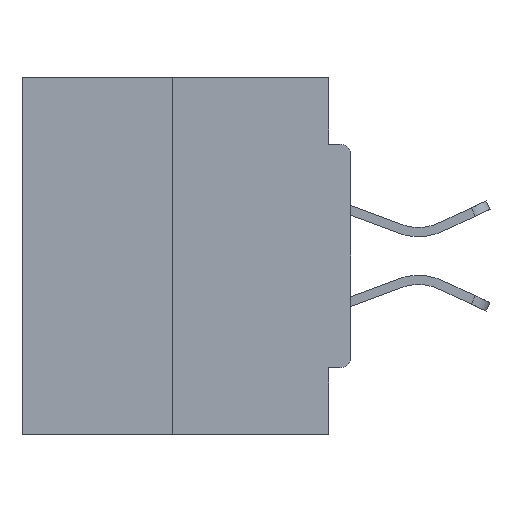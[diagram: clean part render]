
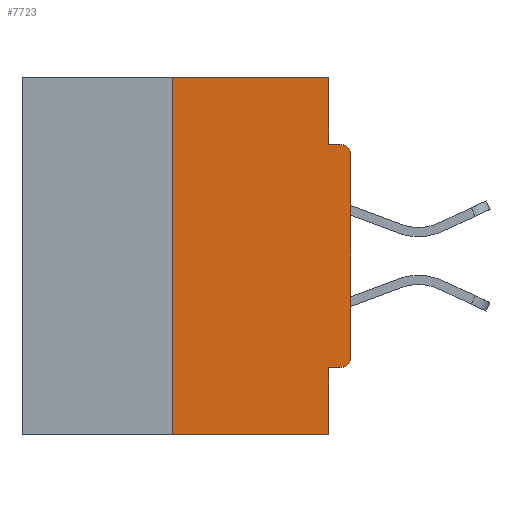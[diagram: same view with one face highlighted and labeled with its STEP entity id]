
A CAD part, left-side view. The second image highlights one B-rep face of the part: STEP entity #7723.
In plain terms, the highlighted planar face has unit normal (-1, 0, 0).
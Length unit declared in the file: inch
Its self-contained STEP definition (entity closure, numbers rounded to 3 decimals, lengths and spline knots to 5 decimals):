
#159 = VERTEX_POINT ( 'NONE', #36421 ) ;
#438 = VERTEX_POINT ( 'NONE', #6405 ) ;
#463 = DIRECTION ( 'NONE',  ( 0., 0., -1. ) ) ;
#654 = CARTESIAN_POINT ( 'NONE',  ( 0., 0., 0. ) ) ;
#776 = LINE ( 'NONE', #13028, #17385 ) ;
#2777 = CARTESIAN_POINT ( 'NONE',  ( 0., 0., -0.0935 ) ) ;
#3005 = ORIENTED_EDGE ( 'NONE', *, *, #11192, .F. ) ;
#3043 = ORIENTED_EDGE ( 'NONE', *, *, #33751, .F. ) ;
#3089 = CARTESIAN_POINT ( 'NONE',  ( 0., 0.031, 0. ) ) ;
#3435 = ORIENTED_EDGE ( 'NONE', *, *, #31251, .F. ) ;
#3451 = DIRECTION ( 'NONE',  ( -1., 0., 0. ) ) ;
#5044 = VECTOR ( 'NONE', #34973, 39.37008 ) ;
#6065 = VECTOR ( 'NONE', #16706, 39.37008 ) ;
#6351 = DIRECTION ( 'NONE',  ( 1., 0., 0. ) ) ;
#6405 = CARTESIAN_POINT ( 'NONE',  ( 0., 0.031, -0.0935 ) ) ;
#6429 = EDGE_CURVE ( 'NONE', #27034, #14101, #776, .T. ) ;
#6594 = AXIS2_PLACEMENT_3D ( 'NONE', #17671, #8720, #463 ) ;
#6656 = ORIENTED_EDGE ( 'NONE', *, *, #34932, .F. ) ;
#6837 = VERTEX_POINT ( 'NONE', #12852 ) ;
#7429 = ORIENTED_EDGE ( 'NONE', *, *, #32899, .T. ) ;
#7723 = ADVANCED_FACE ( 'NONE', ( #20023 ), #23178, .F. ) ;
#7780 = EDGE_CURVE ( 'NONE', #6837, #30905, #22709, .T. ) ;
#8025 = CARTESIAN_POINT ( 'NONE',  ( 0., 0.031, 0. ) ) ;
#8124 = VECTOR ( 'NONE', #19732, 39.37008 ) ;
#8354 = CARTESIAN_POINT ( 'NONE',  ( 0., 0.25, 0. ) ) ;
#8720 = DIRECTION ( 'NONE',  ( -1., 0., 0. ) ) ;
#8802 = CARTESIAN_POINT ( 'NONE',  ( 0., 0.46, -0.5 ) ) ;
#9213 = EDGE_CURVE ( 'NONE', #13541, #30361, #21698, .T. ) ;
#10142 = ORIENTED_EDGE ( 'NONE', *, *, #28367, .F. ) ;
#10775 = CARTESIAN_POINT ( 'NONE',  ( 0., 0.25, 0. ) ) ;
#10821 = EDGE_LOOP ( 'NONE', ( #23040, #6656, #7429, #3435, #3005, #33921, #20419, #21114, #3043, #10142 ) ) ;
#11024 = LINE ( 'NONE', #8802, #32306 ) ;
#11192 = EDGE_CURVE ( 'NONE', #13541, #24240, #19266, .T. ) ;
#11723 = DIRECTION ( 'NONE',  ( 0., 0., -1. ) ) ;
#12223 = CARTESIAN_POINT ( 'NONE',  ( 0., 0.031, -0.5 ) ) ;
#12396 = CARTESIAN_POINT ( 'NONE',  ( 0., 0.015, -0.0935 ) ) ;
#12852 = CARTESIAN_POINT ( 'NONE',  ( 0., 0., -0.1085 ) ) ;
#12979 = CARTESIAN_POINT ( 'NONE',  ( 0., 0.031, -0.4065 ) ) ;
#13028 = CARTESIAN_POINT ( 'NONE',  ( 0., 0.46, 0. ) ) ;
#13541 = VERTEX_POINT ( 'NONE', #21188 ) ;
#14094 = CARTESIAN_POINT ( 'NONE',  ( 0., 0., -0.4065 ) ) ;
#14101 = VERTEX_POINT ( 'NONE', #8025 ) ;
#14108 = LINE ( 'NONE', #2777, #6065 ) ;
#16706 = DIRECTION ( 'NONE',  ( 0., -1., 0. ) ) ;
#17037 = VECTOR ( 'NONE', #35684, 39.37008 ) ;
#17251 = DIRECTION ( 'NONE',  ( 0., -1., 0. ) ) ;
#17385 = VECTOR ( 'NONE', #33639, 39.37008 ) ;
#17671 = CARTESIAN_POINT ( 'NONE',  ( 0., 0.015, -0.1085 ) ) ;
#19266 = LINE ( 'NONE', #14094, #17037 ) ;
#19732 = DIRECTION ( 'NONE',  ( 0., 0., 1. ) ) ;
#20023 = FACE_OUTER_BOUND ( 'NONE', #10821, .T. ) ;
#20419 = ORIENTED_EDGE ( 'NONE', *, *, #22664, .T. ) ;
#20797 = AXIS2_PLACEMENT_3D ( 'NONE', #35104, #6351, #11723 ) ;
#20971 = DIRECTION ( 'NONE',  ( 0., 0., 1. ) ) ;
#21114 = ORIENTED_EDGE ( 'NONE', *, *, #7780, .T. ) ;
#21188 = CARTESIAN_POINT ( 'NONE',  ( 0., 0.015, -0.4065 ) ) ;
#21698 = CIRCLE ( 'NONE', #24425, 0.015 ) ;
#21889 = VECTOR ( 'NONE', #20971, 39.37008 ) ;
#22664 = EDGE_CURVE ( 'NONE', #30361, #6837, #31887, .T. ) ;
#22709 = CIRCLE ( 'NONE', #6594, 0.015 ) ;
#23040 = ORIENTED_EDGE ( 'NONE', *, *, #6429, .F. ) ;
#23178 = PLANE ( 'NONE',  #20797 ) ;
#23322 = VECTOR ( 'NONE', #32589, 39.37008 ) ;
#24173 = VERTEX_POINT ( 'NONE', #27129 ) ;
#24240 = VERTEX_POINT ( 'NONE', #12979 ) ;
#24425 = AXIS2_PLACEMENT_3D ( 'NONE', #34839, #3451, #26453 ) ;
#25134 = LINE ( 'NONE', #12223, #23322 ) ;
#26453 = DIRECTION ( 'NONE',  ( 0., 0., -1. ) ) ;
#27034 = VERTEX_POINT ( 'NONE', #8354 ) ;
#27129 = CARTESIAN_POINT ( 'NONE',  ( 0., 0.031, -0.5 ) ) ;
#27521 = LINE ( 'NONE', #3089, #5044 ) ;
#28367 = EDGE_CURVE ( 'NONE', #14101, #438, #27521, .T. ) ;
#28718 = CARTESIAN_POINT ( 'NONE',  ( 0., 0., -0.3915 ) ) ;
#30361 = VERTEX_POINT ( 'NONE', #28718 ) ;
#30905 = VERTEX_POINT ( 'NONE', #12396 ) ;
#31134 = LINE ( 'NONE', #10775, #8124 ) ;
#31251 = EDGE_CURVE ( 'NONE', #24240, #24173, #25134, .T. ) ;
#31887 = LINE ( 'NONE', #654, #21889 ) ;
#32306 = VECTOR ( 'NONE', #17251, 39.37008 ) ;
#32589 = DIRECTION ( 'NONE',  ( 0., 0., -1. ) ) ;
#32899 = EDGE_CURVE ( 'NONE', #159, #24173, #11024, .T. ) ;
#33639 = DIRECTION ( 'NONE',  ( 0., -1., 0. ) ) ;
#33751 = EDGE_CURVE ( 'NONE', #438, #30905, #14108, .T. ) ;
#33921 = ORIENTED_EDGE ( 'NONE', *, *, #9213, .T. ) ;
#34839 = CARTESIAN_POINT ( 'NONE',  ( 0., 0.015, -0.3915 ) ) ;
#34932 = EDGE_CURVE ( 'NONE', #159, #27034, #31134, .T. ) ;
#34973 = DIRECTION ( 'NONE',  ( 0., 0., -1. ) ) ;
#35104 = CARTESIAN_POINT ( 'NONE',  ( 0., 0.46, 0. ) ) ;
#35684 = DIRECTION ( 'NONE',  ( 0., 1., 0. ) ) ;
#36421 = CARTESIAN_POINT ( 'NONE',  ( 0., 0.25, -0.5 ) ) ;
